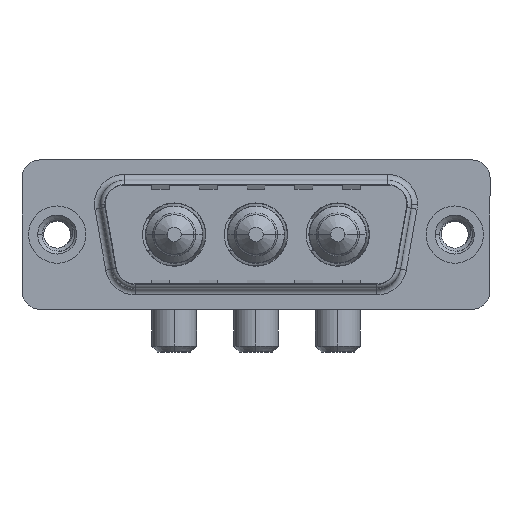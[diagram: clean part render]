
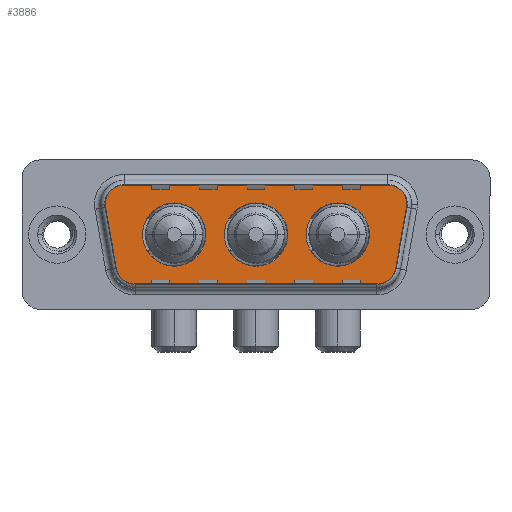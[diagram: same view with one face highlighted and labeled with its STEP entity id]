
A CAD part, top view. The second image highlights one B-rep face of the part: STEP entity #3886.
In plain terms, the highlighted planar face has unit normal (0, 0, 1).
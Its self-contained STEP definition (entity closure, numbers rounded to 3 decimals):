
#273 = DIRECTION ( 'NONE',  ( 0., 0., 1. ) ) ;
#295 = EDGE_CURVE ( 'NONE', #6074, #9929, #5088, .T. ) ;
#326 = CARTESIAN_POINT ( 'NONE',  ( 27.889, 4.9, 0. ) ) ;
#338 = DIRECTION ( 'NONE',  ( 1., 0., 0. ) ) ;
#340 = ORIENTED_EDGE ( 'NONE', *, *, #8777, .T. ) ;
#385 = EDGE_CURVE ( 'NONE', #2379, #11965, #3215, .T. ) ;
#487 = ORIENTED_EDGE ( 'NONE', *, *, #9086, .F. ) ;
#505 = VECTOR ( 'NONE', #2671, 1000. ) ;
#537 = CIRCLE ( 'NONE', #4306, 2.65 ) ;
#688 = DIRECTION ( 'NONE',  ( -1., 0., 0. ) ) ;
#1161 = EDGE_LOOP ( 'NONE', ( #12369, #7743 ) ) ;
#1482 = CIRCLE ( 'NONE', #12120, 2.65 ) ;
#1589 = CARTESIAN_POINT ( 'NONE',  ( 19.3, 0., 0. ) ) ;
#1636 = VECTOR ( 'NONE', #6766, 1000. ) ;
#1761 = VERTEX_POINT ( 'NONE', #2368 ) ;
#1834 = FACE_OUTER_BOUND ( 'NONE', #9028, .T. ) ;
#1853 = CARTESIAN_POINT ( 'NONE',  ( 16.65, 0., 0. ) ) ;
#1998 = AXIS2_PLACEMENT_3D ( 'NONE', #4464, #8697, #8456 ) ;
#2368 = CARTESIAN_POINT ( 'NONE',  ( 5.411, 4.9, 0. ) ) ;
#2379 = VERTEX_POINT ( 'NONE', #11352 ) ;
#2420 = DIRECTION ( 'NONE',  ( 1., 0., 0. ) ) ;
#2454 = EDGE_CURVE ( 'NONE', #11457, #1761, #8618, .T. ) ;
#2471 = DIRECTION ( 'NONE',  ( 0., 0., 1. ) ) ;
#2472 = AXIS2_PLACEMENT_3D ( 'NONE', #10083, #273, #7151 ) ;
#2671 = DIRECTION ( 'NONE',  ( -1., 0., 0. ) ) ;
#2828 = VERTEX_POINT ( 'NONE', #9830 ) ;
#2841 = AXIS2_PLACEMENT_3D ( 'NONE', #8827, #12798, #5948 ) ;
#3215 = CIRCLE ( 'NONE', #10509, 2.65 ) ;
#3268 = EDGE_CURVE ( 'NONE', #2828, #10026, #12829, .T. ) ;
#3309 = CARTESIAN_POINT ( 'NONE',  ( 26.866, -2.9, 0. ) ) ;
#3313 = CARTESIAN_POINT ( 'NONE',  ( 23.5, 0., 0. ) ) ;
#3402 = EDGE_CURVE ( 'NONE', #1761, #6392, #6579, .T. ) ;
#3480 = CARTESIAN_POINT ( 'NONE',  ( 16.65, 0., 0. ) ) ;
#3567 = VERTEX_POINT ( 'NONE', #11292 ) ;
#3612 = ORIENTED_EDGE ( 'NONE', *, *, #7641, .F. ) ;
#3659 = VERTEX_POINT ( 'NONE', #10380 ) ;
#3869 = DIRECTION ( 'NONE',  ( 0., 0., 1. ) ) ;
#3886 = ADVANCED_FACE ( 'NONE', ( #11309, #9805, #11953, #1834 ), #4908, .T. ) ;
#3890 = CARTESIAN_POINT ( 'NONE',  ( 6.434, -4.9, 0. ) ) ;
#4156 = DIRECTION ( 'NONE',  ( 1., 0., 0. ) ) ;
#4294 = EDGE_CURVE ( 'NONE', #12519, #3567, #537, .T. ) ;
#4306 = AXIS2_PLACEMENT_3D ( 'NONE', #6529, #12593, #2420 ) ;
#4367 = CIRCLE ( 'NONE', #2472, 2.65 ) ;
#4464 = CARTESIAN_POINT ( 'NONE',  ( 27.889, 2.9, 0. ) ) ;
#4545 = CARTESIAN_POINT ( 'NONE',  ( 27.889, 2.9, 0. ) ) ;
#4908 = PLANE ( 'NONE',  #11784 ) ;
#4924 = DIRECTION ( 'NONE',  ( 1., 0., 0. ) ) ;
#4970 = AXIS2_PLACEMENT_3D ( 'NONE', #4545, #6449, #688 ) ;
#5024 = CARTESIAN_POINT ( 'NONE',  ( 6.434, -4.9, 0. ) ) ;
#5088 = CIRCLE ( 'NONE', #10099, 2. ) ;
#5128 = DIRECTION ( 'NONE',  ( 0., 0., 1. ) ) ;
#5476 = ORIENTED_EDGE ( 'NONE', *, *, #8845, .F. ) ;
#5839 = DIRECTION ( 'NONE',  ( 0., 0., 1. ) ) ;
#5948 = DIRECTION ( 'NONE',  ( 1., 0., 0. ) ) ;
#6074 = VERTEX_POINT ( 'NONE', #7346 ) ;
#6392 = VERTEX_POINT ( 'NONE', #9325 ) ;
#6449 = DIRECTION ( 'NONE',  ( 0., 0., 1. ) ) ;
#6472 = ORIENTED_EDGE ( 'NONE', *, *, #295, .T. ) ;
#6495 = CARTESIAN_POINT ( 'NONE',  ( 29.889, 2.9, 0. ) ) ;
#6508 = EDGE_CURVE ( 'NONE', #10026, #11457, #10601, .T. ) ;
#6516 = DIRECTION ( 'NONE',  ( 0., 0., 1. ) ) ;
#6529 = CARTESIAN_POINT ( 'NONE',  ( 9.8, 0., 0. ) ) ;
#6579 = CIRCLE ( 'NONE', #2841, 2. ) ;
#6631 = CARTESIAN_POINT ( 'NONE',  ( 7.15, 0., 0. ) ) ;
#6766 = DIRECTION ( 'NONE',  ( 1., 0., 0. ) ) ;
#6885 = AXIS2_PLACEMENT_3D ( 'NONE', #3309, #5128, #4156 ) ;
#7094 = AXIS2_PLACEMENT_3D ( 'NONE', #3480, #9354, #338 ) ;
#7151 = DIRECTION ( 'NONE',  ( 1., 0., 0. ) ) ;
#7292 = VERTEX_POINT ( 'NONE', #11971 ) ;
#7300 = LINE ( 'NONE', #8041, #11063 ) ;
#7346 = CARTESIAN_POINT ( 'NONE',  ( 4.464, -3.247, 0. ) ) ;
#7503 = CARTESIAN_POINT ( 'NONE',  ( 23.5, 0., 0. ) ) ;
#7641 = EDGE_CURVE ( 'NONE', #3567, #12519, #4367, .T. ) ;
#7743 = ORIENTED_EDGE ( 'NONE', *, *, #385, .F. ) ;
#7920 = ORIENTED_EDGE ( 'NONE', *, *, #9840, .T. ) ;
#7925 = CIRCLE ( 'NONE', #6885, 2. ) ;
#8041 = CARTESIAN_POINT ( 'NONE',  ( 29.859, 2.553, 0. ) ) ;
#8057 = LINE ( 'NONE', #9943, #8351 ) ;
#8351 = VECTOR ( 'NONE', #10979, 1000. ) ;
#8417 = DIRECTION ( 'NONE',  ( -1., 0., 0. ) ) ;
#8456 = DIRECTION ( 'NONE',  ( -1., 0., 0. ) ) ;
#8581 = EDGE_CURVE ( 'NONE', #7292, #11806, #7925, .T. ) ;
#8618 = LINE ( 'NONE', #9594, #505 ) ;
#8697 = DIRECTION ( 'NONE',  ( 0., 0., 1. ) ) ;
#8764 = DIRECTION ( 'NONE',  ( 1., 0., 0. ) ) ;
#8771 = EDGE_LOOP ( 'NONE', ( #487, #5476 ) ) ;
#8777 = EDGE_CURVE ( 'NONE', #9929, #7292, #11637, .T. ) ;
#8827 = CARTESIAN_POINT ( 'NONE',  ( 5.411, 2.9, 0. ) ) ;
#8845 = EDGE_CURVE ( 'NONE', #3659, #10057, #11244, .T. ) ;
#8960 = CARTESIAN_POINT ( 'NONE',  ( 26.866, -2.9, 0. ) ) ;
#9028 = EDGE_LOOP ( 'NONE', ( #9091, #7920, #9972, #10821, #12835, #12173, #9329, #6472, #340 ) ) ;
#9086 = EDGE_CURVE ( 'NONE', #10057, #3659, #11250, .T. ) ;
#9091 = ORIENTED_EDGE ( 'NONE', *, *, #8581, .T. ) ;
#9204 = EDGE_LOOP ( 'NONE', ( #3612, #10857 ) ) ;
#9325 = CARTESIAN_POINT ( 'NONE',  ( 3.441, 2.553, 0. ) ) ;
#9329 = ORIENTED_EDGE ( 'NONE', *, *, #9451, .T. ) ;
#9354 = DIRECTION ( 'NONE',  ( 0., 0., 1. ) ) ;
#9451 = EDGE_CURVE ( 'NONE', #6392, #6074, #8057, .T. ) ;
#9594 = CARTESIAN_POINT ( 'NONE',  ( 5.411, 4.9, 0. ) ) ;
#9805 = FACE_BOUND ( 'NONE', #1161, .T. ) ;
#9830 = CARTESIAN_POINT ( 'NONE',  ( 29.859, 2.553, 0. ) ) ;
#9840 = EDGE_CURVE ( 'NONE', #11806, #2828, #7300, .T. ) ;
#9929 = VERTEX_POINT ( 'NONE', #5024 ) ;
#9943 = CARTESIAN_POINT ( 'NONE',  ( 3.441, 2.553, 0. ) ) ;
#9972 = ORIENTED_EDGE ( 'NONE', *, *, #3268, .T. ) ;
#10026 = VERTEX_POINT ( 'NONE', #6495 ) ;
#10057 = VERTEX_POINT ( 'NONE', #1589 ) ;
#10083 = CARTESIAN_POINT ( 'NONE',  ( 9.8, 0., 0. ) ) ;
#10099 = AXIS2_PLACEMENT_3D ( 'NONE', #12797, #2471, #8417 ) ;
#10208 = AXIS2_PLACEMENT_3D ( 'NONE', #1853, #5839, #4924 ) ;
#10229 = DIRECTION ( 'NONE',  ( 0.174, 0.985, 0. ) ) ;
#10311 = CARTESIAN_POINT ( 'NONE',  ( 26.15, 0., 0. ) ) ;
#10380 = CARTESIAN_POINT ( 'NONE',  ( 14., 0., 0. ) ) ;
#10509 = AXIS2_PLACEMENT_3D ( 'NONE', #7503, #6516, #12516 ) ;
#10601 = CIRCLE ( 'NONE', #4970, 2. ) ;
#10821 = ORIENTED_EDGE ( 'NONE', *, *, #6508, .T. ) ;
#10857 = ORIENTED_EDGE ( 'NONE', *, *, #4294, .F. ) ;
#10970 = CARTESIAN_POINT ( 'NONE',  ( 28.836, -3.247, 0. ) ) ;
#10979 = DIRECTION ( 'NONE',  ( 0.174, -0.985, 0. ) ) ;
#11011 = EDGE_CURVE ( 'NONE', #11965, #2379, #1482, .T. ) ;
#11063 = VECTOR ( 'NONE', #10229, 1000. ) ;
#11244 = CIRCLE ( 'NONE', #10208, 2.65 ) ;
#11250 = CIRCLE ( 'NONE', #7094, 2.65 ) ;
#11269 = DIRECTION ( 'NONE',  ( 0., 0., 1. ) ) ;
#11292 = CARTESIAN_POINT ( 'NONE',  ( 12.45, 0., 0. ) ) ;
#11309 = FACE_BOUND ( 'NONE', #8771, .T. ) ;
#11331 = DIRECTION ( 'NONE',  ( 1., 0., 0. ) ) ;
#11352 = CARTESIAN_POINT ( 'NONE',  ( 20.85, 0., 0. ) ) ;
#11457 = VERTEX_POINT ( 'NONE', #326 ) ;
#11637 = LINE ( 'NONE', #3890, #1636 ) ;
#11784 = AXIS2_PLACEMENT_3D ( 'NONE', #8960, #3869, #8764 ) ;
#11806 = VERTEX_POINT ( 'NONE', #10970 ) ;
#11953 = FACE_BOUND ( 'NONE', #9204, .T. ) ;
#11965 = VERTEX_POINT ( 'NONE', #10311 ) ;
#11971 = CARTESIAN_POINT ( 'NONE',  ( 26.866, -4.9, 0. ) ) ;
#12120 = AXIS2_PLACEMENT_3D ( 'NONE', #3313, #11269, #11331 ) ;
#12173 = ORIENTED_EDGE ( 'NONE', *, *, #3402, .T. ) ;
#12369 = ORIENTED_EDGE ( 'NONE', *, *, #11011, .F. ) ;
#12516 = DIRECTION ( 'NONE',  ( 1., 0., 0. ) ) ;
#12519 = VERTEX_POINT ( 'NONE', #6631 ) ;
#12593 = DIRECTION ( 'NONE',  ( 0., 0., 1. ) ) ;
#12797 = CARTESIAN_POINT ( 'NONE',  ( 6.434, -2.9, 0. ) ) ;
#12798 = DIRECTION ( 'NONE',  ( 0., 0., 1. ) ) ;
#12829 = CIRCLE ( 'NONE', #1998, 2. ) ;
#12835 = ORIENTED_EDGE ( 'NONE', *, *, #2454, .T. ) ;
